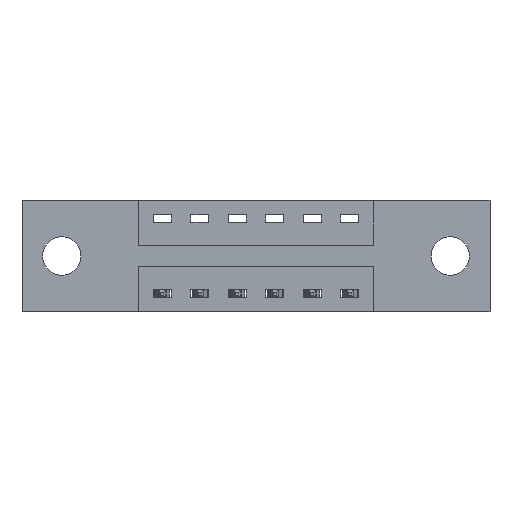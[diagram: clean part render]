
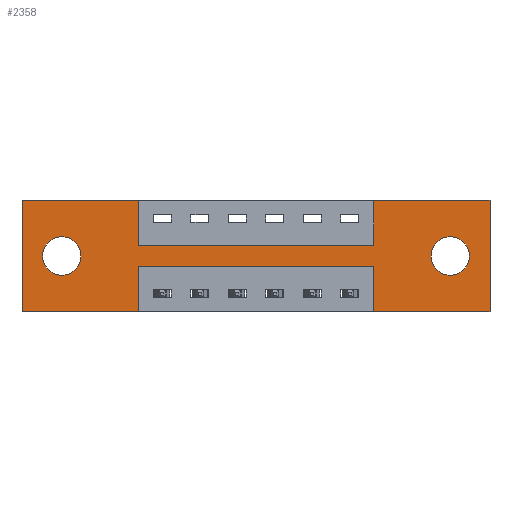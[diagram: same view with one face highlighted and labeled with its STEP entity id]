
A CAD part, front view. The second image highlights one B-rep face of the part: STEP entity #2358.
In plain terms, the highlighted planar face has unit normal (0, -1, 0).
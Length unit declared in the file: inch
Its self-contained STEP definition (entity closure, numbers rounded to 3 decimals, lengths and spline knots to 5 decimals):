
#7 = ORIENTED_EDGE ( 'NONE', *, *, #4430, .F. ) ;
#71 = VECTOR ( 'NONE', #1446, 39.37008 ) ;
#98 = EDGE_CURVE ( 'NONE', #816, #7506, #8371, .T. ) ;
#181 = DIRECTION ( 'NONE',  ( 1., 0., 0. ) ) ;
#199 = AXIS2_PLACEMENT_3D ( 'NONE', #8374, #4445, #493 ) ;
#311 = VECTOR ( 'NONE', #1024, 39.37008 ) ;
#329 = CARTESIAN_POINT ( 'NONE',  ( 0.3875, 0., -0.15 ) ) ;
#493 = DIRECTION ( 'NONE',  ( 0., 0., -1. ) ) ;
#560 = LINE ( 'NONE', #5355, #3877 ) ;
#785 = VERTEX_POINT ( 'NONE', #3994 ) ;
#816 = VERTEX_POINT ( 'NONE', #1317 ) ;
#875 = DIRECTION ( 'NONE',  ( -1., 0., 0. ) ) ;
#955 = DIRECTION ( 'NONE',  ( 0., 1., 0. ) ) ;
#1024 = DIRECTION ( 'NONE',  ( 1., 0., 0. ) ) ;
#1108 = LINE ( 'NONE', #2841, #4797 ) ;
#1260 = CARTESIAN_POINT ( 'NONE',  ( 0., 0., -0.37 ) ) ;
#1287 = LINE ( 'NONE', #7662, #6314 ) ;
#1309 = VERTEX_POINT ( 'NONE', #1372 ) ;
#1317 = CARTESIAN_POINT ( 'NONE',  ( 0.3875, 0., -0.22 ) ) ;
#1351 = EDGE_CURVE ( 'NONE', #785, #6469, #1287, .T. ) ;
#1372 = CARTESIAN_POINT ( 'NONE',  ( 1.1725, 0., -0.15 ) ) ;
#1409 = ORIENTED_EDGE ( 'NONE', *, *, #2406, .F. ) ;
#1446 = DIRECTION ( 'NONE',  ( 0., 0., 1. ) ) ;
#1624 = VERTEX_POINT ( 'NONE', #2526 ) ;
#1741 = EDGE_CURVE ( 'NONE', #6537, #5339, #1814, .T. ) ;
#1814 = LINE ( 'NONE', #7335, #7733 ) ;
#1874 = CARTESIAN_POINT ( 'NONE',  ( 0.3875, 0., -0.37 ) ) ;
#1883 = EDGE_CURVE ( 'NONE', #1309, #8312, #560, .T. ) ;
#1896 = DIRECTION ( 'NONE',  ( 0., -1., 0. ) ) ;
#1972 = VECTOR ( 'NONE', #3452, 39.37008 ) ;
#1978 = CARTESIAN_POINT ( 'NONE',  ( 1.1725, 0., 0. ) ) ;
#2036 = ORIENTED_EDGE ( 'NONE', *, *, #3387, .F. ) ;
#2099 = LINE ( 'NONE', #329, #311 ) ;
#2109 = FACE_BOUND ( 'NONE', #3189, .T. ) ;
#2144 = EDGE_CURVE ( 'NONE', #6432, #5261, #5296, .T. ) ;
#2346 = ORIENTED_EDGE ( 'NONE', *, *, #5271, .T. ) ;
#2358 = ADVANCED_FACE ( 'NONE', ( #2109, #4071, #7520 ), #8459, .T. ) ;
#2376 = EDGE_CURVE ( 'NONE', #7506, #3659, #5397, .T. ) ;
#2379 = CARTESIAN_POINT ( 'NONE',  ( 0.3875, 0., -0.15 ) ) ;
#2406 = EDGE_CURVE ( 'NONE', #4102, #5817, #6905, .T. ) ;
#2453 = EDGE_CURVE ( 'NONE', #5261, #6432, #8271, .T. ) ;
#2526 = CARTESIAN_POINT ( 'NONE',  ( 1.4275, 0., -0.121 ) ) ;
#2763 = ORIENTED_EDGE ( 'NONE', *, *, #98, .F. ) ;
#2841 = CARTESIAN_POINT ( 'NONE',  ( 0., 0., -0.37 ) ) ;
#2893 = EDGE_CURVE ( 'NONE', #7416, #1309, #2099, .T. ) ;
#2964 = ORIENTED_EDGE ( 'NONE', *, *, #7913, .F. ) ;
#3157 = LINE ( 'NONE', #3770, #4894 ) ;
#3189 = EDGE_LOOP ( 'NONE', ( #7324, #2346 ) ) ;
#3365 = ORIENTED_EDGE ( 'NONE', *, *, #1883, .F. ) ;
#3387 = EDGE_CURVE ( 'NONE', #3659, #6537, #3424, .T. ) ;
#3424 = LINE ( 'NONE', #6678, #71 ) ;
#3425 = AXIS2_PLACEMENT_3D ( 'NONE', #5834, #1896, #6481 ) ;
#3452 = DIRECTION ( 'NONE',  ( 1., 0., 0. ) ) ;
#3536 = CARTESIAN_POINT ( 'NONE',  ( 0.1325, 0., -0.249 ) ) ;
#3644 = VECTOR ( 'NONE', #8521, 39.37008 ) ;
#3659 = VERTEX_POINT ( 'NONE', #6267 ) ;
#3682 = CARTESIAN_POINT ( 'NONE',  ( 0.1325, 0., -0.185 ) ) ;
#3696 = EDGE_LOOP ( 'NONE', ( #2763, #2964, #6441, #8201, #1409, #8407, #3365, #6822, #7, #7040, #2036, #5526 ) ) ;
#3770 = CARTESIAN_POINT ( 'NONE',  ( 0.3875, 0., -0.22 ) ) ;
#3877 = VECTOR ( 'NONE', #7996, 39.37008 ) ;
#3896 = DIRECTION ( 'NONE',  ( 0., 0., -1. ) ) ;
#3928 = LINE ( 'NONE', #6384, #1972 ) ;
#3964 = CARTESIAN_POINT ( 'NONE',  ( 1.1725, 0., -0.22 ) ) ;
#3968 = CARTESIAN_POINT ( 'NONE',  ( 0.1325, 0., -0.185 ) ) ;
#3994 = CARTESIAN_POINT ( 'NONE',  ( 1.1725, 0., -0.37 ) ) ;
#4071 = FACE_BOUND ( 'NONE', #8505, .T. ) ;
#4102 = VERTEX_POINT ( 'NONE', #4147 ) ;
#4147 = CARTESIAN_POINT ( 'NONE',  ( 1.56, 0., 0. ) ) ;
#4193 = VERTEX_POINT ( 'NONE', #4234 ) ;
#4234 = CARTESIAN_POINT ( 'NONE',  ( 1.4275, 0., -0.249 ) ) ;
#4346 = DIRECTION ( 'NONE',  ( 0., 0., 1. ) ) ;
#4399 = DIRECTION ( 'NONE',  ( -1., 0., 0. ) ) ;
#4430 = EDGE_CURVE ( 'NONE', #5339, #7416, #6485, .T. ) ;
#4445 = DIRECTION ( 'NONE',  ( 0., 1., 0. ) ) ;
#4564 = CARTESIAN_POINT ( 'NONE',  ( 1.56, 0., 0. ) ) ;
#4624 = DIRECTION ( 'NONE',  ( 0., 0., 1. ) ) ;
#4797 = VECTOR ( 'NONE', #875, 39.37008 ) ;
#4892 = CARTESIAN_POINT ( 'NONE',  ( 1.4275, 0., -0.185 ) ) ;
#4894 = VECTOR ( 'NONE', #4399, 39.37008 ) ;
#4983 = VECTOR ( 'NONE', #6532, 39.37008 ) ;
#5102 = EDGE_CURVE ( 'NONE', #1624, #4193, #5872, .T. ) ;
#5121 = EDGE_CURVE ( 'NONE', #8312, #4102, #3928, .T. ) ;
#5191 = AXIS2_PLACEMENT_3D ( 'NONE', #3968, #8571, #4624 ) ;
#5261 = VERTEX_POINT ( 'NONE', #3536 ) ;
#5271 = EDGE_CURVE ( 'NONE', #4193, #1624, #6370, .T. ) ;
#5296 = CIRCLE ( 'NONE', #6651, 0.064 ) ;
#5339 = VERTEX_POINT ( 'NONE', #7563 ) ;
#5355 = CARTESIAN_POINT ( 'NONE',  ( 1.1725, 0., 0. ) ) ;
#5397 = LINE ( 'NONE', #1260, #3644 ) ;
#5526 = ORIENTED_EDGE ( 'NONE', *, *, #2376, .F. ) ;
#5557 = DIRECTION ( 'NONE',  ( 0., 0., -1. ) ) ;
#5817 = VERTEX_POINT ( 'NONE', #8014 ) ;
#5834 = CARTESIAN_POINT ( 'NONE',  ( 0., 0., -0.37 ) ) ;
#5872 = CIRCLE ( 'NONE', #199, 0.064 ) ;
#6032 = ORIENTED_EDGE ( 'NONE', *, *, #2453, .T. ) ;
#6086 = AXIS2_PLACEMENT_3D ( 'NONE', #4892, #955, #5557 ) ;
#6267 = CARTESIAN_POINT ( 'NONE',  ( 0., 0., -0.37 ) ) ;
#6314 = VECTOR ( 'NONE', #7609, 39.37008 ) ;
#6370 = CIRCLE ( 'NONE', #6086, 0.064 ) ;
#6384 = CARTESIAN_POINT ( 'NONE',  ( 0., 0., 0. ) ) ;
#6432 = VERTEX_POINT ( 'NONE', #7824 ) ;
#6441 = ORIENTED_EDGE ( 'NONE', *, *, #1351, .F. ) ;
#6469 = VERTEX_POINT ( 'NONE', #3964 ) ;
#6481 = DIRECTION ( 'NONE',  ( 0., 0., -1. ) ) ;
#6485 = LINE ( 'NONE', #7807, #7818 ) ;
#6532 = DIRECTION ( 'NONE',  ( 0., 0., -1. ) ) ;
#6537 = VERTEX_POINT ( 'NONE', #7384 ) ;
#6605 = VECTOR ( 'NONE', #7345, 39.37008 ) ;
#6651 = AXIS2_PLACEMENT_3D ( 'NONE', #3682, #8275, #4346 ) ;
#6678 = CARTESIAN_POINT ( 'NONE',  ( 0., 0., 0. ) ) ;
#6822 = ORIENTED_EDGE ( 'NONE', *, *, #2893, .F. ) ;
#6905 = LINE ( 'NONE', #4564, #4983 ) ;
#7040 = ORIENTED_EDGE ( 'NONE', *, *, #1741, .F. ) ;
#7269 = EDGE_CURVE ( 'NONE', #5817, #785, #1108, .T. ) ;
#7324 = ORIENTED_EDGE ( 'NONE', *, *, #5102, .T. ) ;
#7335 = CARTESIAN_POINT ( 'NONE',  ( 0., 0., 0. ) ) ;
#7345 = DIRECTION ( 'NONE',  ( 0., 0., -1. ) ) ;
#7384 = CARTESIAN_POINT ( 'NONE',  ( 0., 0., 0. ) ) ;
#7416 = VERTEX_POINT ( 'NONE', #2379 ) ;
#7506 = VERTEX_POINT ( 'NONE', #1874 ) ;
#7520 = FACE_OUTER_BOUND ( 'NONE', #3696, .T. ) ;
#7548 = ORIENTED_EDGE ( 'NONE', *, *, #2144, .T. ) ;
#7563 = CARTESIAN_POINT ( 'NONE',  ( 0.3875, 0., 0. ) ) ;
#7609 = DIRECTION ( 'NONE',  ( 0., 0., 1. ) ) ;
#7662 = CARTESIAN_POINT ( 'NONE',  ( 1.1725, 0., -0.37 ) ) ;
#7733 = VECTOR ( 'NONE', #181, 39.37008 ) ;
#7807 = CARTESIAN_POINT ( 'NONE',  ( 0.3875, 0., 0. ) ) ;
#7818 = VECTOR ( 'NONE', #3896, 39.37008 ) ;
#7824 = CARTESIAN_POINT ( 'NONE',  ( 0.1325, 0., -0.121 ) ) ;
#7913 = EDGE_CURVE ( 'NONE', #6469, #816, #3157, .T. ) ;
#7996 = DIRECTION ( 'NONE',  ( 0., 0., 1. ) ) ;
#8014 = CARTESIAN_POINT ( 'NONE',  ( 1.56, 0., -0.37 ) ) ;
#8201 = ORIENTED_EDGE ( 'NONE', *, *, #7269, .F. ) ;
#8271 = CIRCLE ( 'NONE', #5191, 0.064 ) ;
#8275 = DIRECTION ( 'NONE',  ( 0., 1., 0. ) ) ;
#8312 = VERTEX_POINT ( 'NONE', #1978 ) ;
#8314 = CARTESIAN_POINT ( 'NONE',  ( 0.3875, 0., -0.37 ) ) ;
#8371 = LINE ( 'NONE', #8314, #6605 ) ;
#8374 = CARTESIAN_POINT ( 'NONE',  ( 1.4275, 0., -0.185 ) ) ;
#8407 = ORIENTED_EDGE ( 'NONE', *, *, #5121, .F. ) ;
#8459 = PLANE ( 'NONE',  #3425 ) ;
#8505 = EDGE_LOOP ( 'NONE', ( #7548, #6032 ) ) ;
#8521 = DIRECTION ( 'NONE',  ( -1., 0., 0. ) ) ;
#8571 = DIRECTION ( 'NONE',  ( 0., 1., 0. ) ) ;
